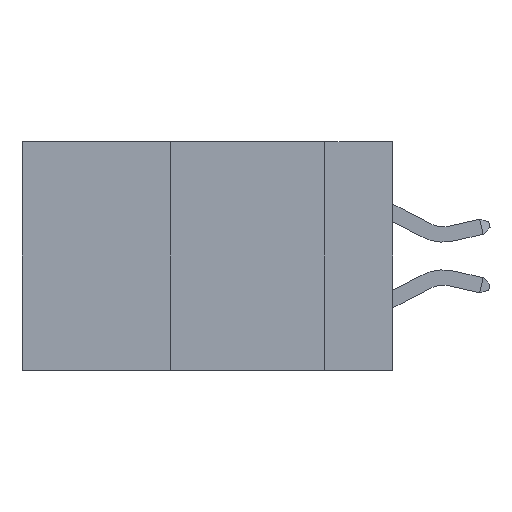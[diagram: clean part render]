
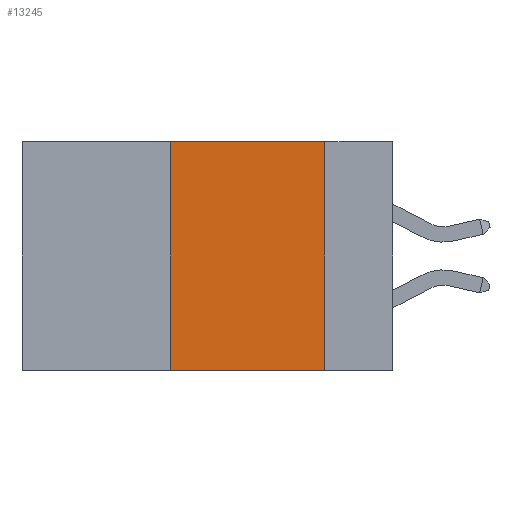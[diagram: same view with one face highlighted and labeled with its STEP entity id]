
A CAD part, left-side view. The second image highlights one B-rep face of the part: STEP entity #13245.
In plain terms, the highlighted planar face has unit normal (-1, 0, 0).
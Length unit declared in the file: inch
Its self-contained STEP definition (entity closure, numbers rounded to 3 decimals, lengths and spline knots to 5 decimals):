
#376 = VERTEX_POINT ( 'NONE', #1894 ) ;
#1090 = LINE ( 'NONE', #4128, #10251 ) ;
#1307 = EDGE_CURVE ( 'NONE', #11556, #7592, #8556, .T. ) ;
#1363 = DIRECTION ( 'NONE',  ( 1., 0., 0. ) ) ;
#1427 = PLANE ( 'NONE',  #8955 ) ;
#1894 = CARTESIAN_POINT ( 'NONE',  ( 0., 0.11, -0.37 ) ) ;
#2268 = CARTESIAN_POINT ( 'NONE',  ( 0., 0.36, 0. ) ) ;
#3159 = DIRECTION ( 'NONE',  ( 0., -1., 0. ) ) ;
#3250 = CARTESIAN_POINT ( 'NONE',  ( 0., 0.36, 0. ) ) ;
#3778 = EDGE_CURVE ( 'NONE', #6728, #376, #13452, .T. ) ;
#4128 = CARTESIAN_POINT ( 'NONE',  ( 0., 0.6, 0. ) ) ;
#4316 = FACE_OUTER_BOUND ( 'NONE', #9611, .T. ) ;
#4523 = DIRECTION ( 'NONE',  ( 0., 0., -1. ) ) ;
#4675 = DIRECTION ( 'NONE',  ( 0., -1., 0. ) ) ;
#5319 = CARTESIAN_POINT ( 'NONE',  ( 0., 0.11, 0. ) ) ;
#5887 = CARTESIAN_POINT ( 'NONE',  ( 0., 0.11, 0. ) ) ;
#6391 = VECTOR ( 'NONE', #7652, 39.37008 ) ;
#6575 = ORIENTED_EDGE ( 'NONE', *, *, #3778, .F. ) ;
#6728 = VERTEX_POINT ( 'NONE', #5319 ) ;
#6927 = CARTESIAN_POINT ( 'NONE',  ( 0., 0.6, -0.37 ) ) ;
#7592 = VERTEX_POINT ( 'NONE', #2268 ) ;
#7652 = DIRECTION ( 'NONE',  ( 0., 0., 1. ) ) ;
#8305 = DIRECTION ( 'NONE',  ( 0., 0., -1. ) ) ;
#8447 = CARTESIAN_POINT ( 'NONE',  ( 0., 0.6, 0. ) ) ;
#8556 = LINE ( 'NONE', #3250, #6391 ) ;
#8725 = VECTOR ( 'NONE', #4675, 39.37008 ) ;
#8955 = AXIS2_PLACEMENT_3D ( 'NONE', #8447, #1363, #4523 ) ;
#9611 = EDGE_LOOP ( 'NONE', ( #6575, #10549, #11388, #12407 ) ) ;
#10251 = VECTOR ( 'NONE', #3159, 39.37008 ) ;
#10549 = ORIENTED_EDGE ( 'NONE', *, *, #11295, .F. ) ;
#11295 = EDGE_CURVE ( 'NONE', #7592, #6728, #1090, .T. ) ;
#11388 = ORIENTED_EDGE ( 'NONE', *, *, #1307, .F. ) ;
#11556 = VERTEX_POINT ( 'NONE', #13142 ) ;
#12239 = LINE ( 'NONE', #6927, #8725 ) ;
#12407 = ORIENTED_EDGE ( 'NONE', *, *, #12932, .T. ) ;
#12868 = VECTOR ( 'NONE', #8305, 39.37008 ) ;
#12932 = EDGE_CURVE ( 'NONE', #11556, #376, #12239, .T. ) ;
#13142 = CARTESIAN_POINT ( 'NONE',  ( 0., 0.36, -0.37 ) ) ;
#13245 = ADVANCED_FACE ( 'NONE', ( #4316 ), #1427, .F. ) ;
#13452 = LINE ( 'NONE', #5887, #12868 ) ;
